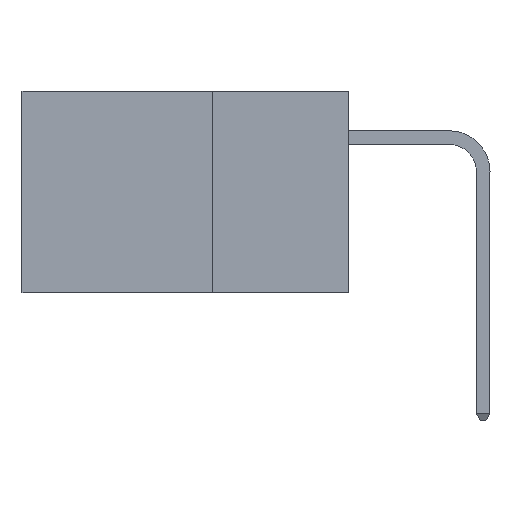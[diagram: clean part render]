
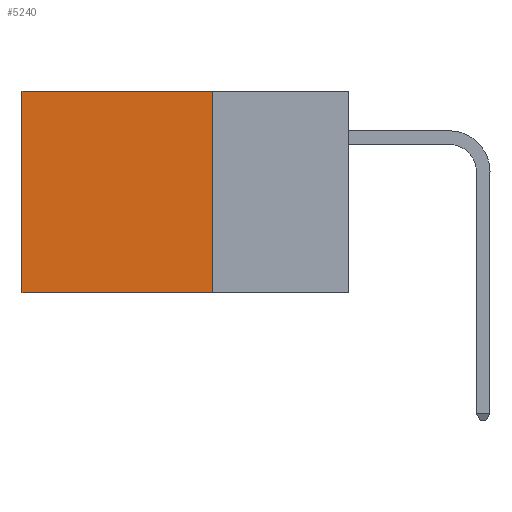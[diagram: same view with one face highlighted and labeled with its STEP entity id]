
A CAD part, left-side view. The second image highlights one B-rep face of the part: STEP entity #5240.
In plain terms, the highlighted planar face has unit normal (-1, 0, 0).
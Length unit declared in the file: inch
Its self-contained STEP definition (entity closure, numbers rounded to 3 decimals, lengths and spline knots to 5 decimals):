
#552 = DIRECTION ( 'NONE',  ( 0., 0., -1. ) ) ;
#722 = FACE_OUTER_BOUND ( 'NONE', #8021, .T. ) ;
#1354 = DIRECTION ( 'NONE',  ( 0., 0., -1. ) ) ;
#1375 = DIRECTION ( 'NONE',  ( 1., 0., 0. ) ) ;
#1684 = PLANE ( 'NONE',  #6131 ) ;
#1888 = VECTOR ( 'NONE', #552, 39.37008 ) ;
#1952 = CARTESIAN_POINT ( 'NONE',  ( 0.2875, 0.25, 0. ) ) ;
#2209 = VECTOR ( 'NONE', #14551, 39.37008 ) ;
#2281 = VERTEX_POINT ( 'NONE', #17341 ) ;
#2524 = LINE ( 'NONE', #12086, #16946 ) ;
#2981 = CARTESIAN_POINT ( 'NONE',  ( 0.2875, 0.25, 0. ) ) ;
#3625 = LINE ( 'NONE', #9207, #10912 ) ;
#4623 = ORIENTED_EDGE ( 'NONE', *, *, #16551, .T. ) ;
#5240 = ADVANCED_FACE ( 'NONE', ( #722 ), #1684, .F. ) ;
#6131 = AXIS2_PLACEMENT_3D ( 'NONE', #1952, #1375, #1354 ) ;
#6350 = EDGE_CURVE ( 'NONE', #2281, #15383, #17228, .T. ) ;
#8021 = EDGE_LOOP ( 'NONE', ( #12752, #15225, #8977, #4623 ) ) ;
#8977 = ORIENTED_EDGE ( 'NONE', *, *, #9667, .F. ) ;
#9189 = VERTEX_POINT ( 'NONE', #13533 ) ;
#9207 = CARTESIAN_POINT ( 'NONE',  ( 0.2875, 0.25, -0.37 ) ) ;
#9477 = CARTESIAN_POINT ( 'NONE',  ( 0.2875, 0.6, 0. ) ) ;
#9667 = EDGE_CURVE ( 'NONE', #11203, #9189, #17516, .T. ) ;
#10912 = VECTOR ( 'NONE', #14965, 39.37008 ) ;
#11203 = VERTEX_POINT ( 'NONE', #16770 ) ;
#12086 = CARTESIAN_POINT ( 'NONE',  ( 0.2875, 0.25, 0. ) ) ;
#12509 = EDGE_CURVE ( 'NONE', #9189, #15383, #3625, .T. ) ;
#12752 = ORIENTED_EDGE ( 'NONE', *, *, #6350, .T. ) ;
#13512 = DIRECTION ( 'NONE',  ( 0., 1., 0. ) ) ;
#13533 = CARTESIAN_POINT ( 'NONE',  ( 0.2875, 0.25, -0.37 ) ) ;
#14551 = DIRECTION ( 'NONE',  ( 0., 0., -1. ) ) ;
#14965 = DIRECTION ( 'NONE',  ( 0., 1., 0. ) ) ;
#15194 = CARTESIAN_POINT ( 'NONE',  ( 0.2875, 0.6, -0.37 ) ) ;
#15225 = ORIENTED_EDGE ( 'NONE', *, *, #12509, .F. ) ;
#15383 = VERTEX_POINT ( 'NONE', #15194 ) ;
#16551 = EDGE_CURVE ( 'NONE', #11203, #2281, #2524, .T. ) ;
#16770 = CARTESIAN_POINT ( 'NONE',  ( 0.2875, 0.25, 0. ) ) ;
#16946 = VECTOR ( 'NONE', #13512, 39.37008 ) ;
#17228 = LINE ( 'NONE', #9477, #1888 ) ;
#17341 = CARTESIAN_POINT ( 'NONE',  ( 0.2875, 0.6, 0. ) ) ;
#17516 = LINE ( 'NONE', #2981, #2209 ) ;
